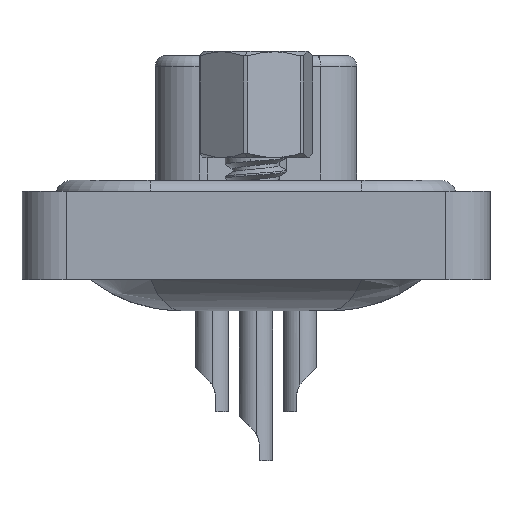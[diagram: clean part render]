
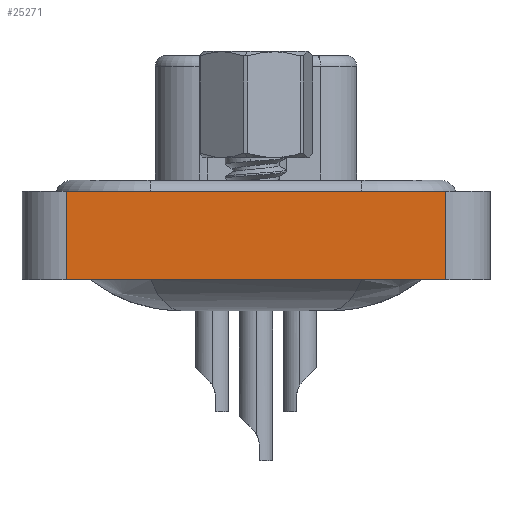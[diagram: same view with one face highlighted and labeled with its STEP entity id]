
A CAD part, left-side view. The second image highlights one B-rep face of the part: STEP entity #25271.
In plain terms, the highlighted planar face has unit normal (-1, 0, 0).
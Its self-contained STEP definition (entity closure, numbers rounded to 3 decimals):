
#2920 = AXIS2_PLACEMENT_3D ( 'NONE', #29742, #21012, #5306 ) ;
#4125 = VECTOR ( 'NONE', #22422, 1000. ) ;
#4745 = EDGE_CURVE ( 'NONE', #5199, #23662, #16815, .T. ) ;
#4768 = PLANE ( 'NONE',  #2920 ) ;
#5199 = VERTEX_POINT ( 'NONE', #11238 ) ;
#5306 = DIRECTION ( 'NONE',  ( 0., 0., 1. ) ) ;
#5752 = VECTOR ( 'NONE', #29520, 1000. ) ;
#6194 = DIRECTION ( 'NONE',  ( 0., 0., 1. ) ) ;
#6858 = ORIENTED_EDGE ( 'NONE', *, *, #12142, .T. ) ;
#8749 = CARTESIAN_POINT ( 'NONE',  ( -7.35, -8.55, 0.4 ) ) ;
#10289 = ORIENTED_EDGE ( 'NONE', *, *, #4745, .F. ) ;
#11238 = CARTESIAN_POINT ( 'NONE',  ( -7.35, 8.55, 0.4 ) ) ;
#12111 = CARTESIAN_POINT ( 'NONE',  ( -7.35, -8.55, -3.6 ) ) ;
#12142 = EDGE_CURVE ( 'NONE', #22488, #22613, #28128, .T. ) ;
#13203 = LINE ( 'NONE', #24951, #16382 ) ;
#13950 = CARTESIAN_POINT ( 'NONE',  ( -7.35, -8.55, 0.4 ) ) ;
#16382 = VECTOR ( 'NONE', #6194, 1000. ) ;
#16497 = EDGE_CURVE ( 'NONE', #22613, #23662, #18637, .T. ) ;
#16815 = LINE ( 'NONE', #13950, #32760 ) ;
#18637 = LINE ( 'NONE', #27011, #5752 ) ;
#20130 = ORIENTED_EDGE ( 'NONE', *, *, #16497, .T. ) ;
#21012 = DIRECTION ( 'NONE',  ( -1., 0., 0. ) ) ;
#22422 = DIRECTION ( 'NONE',  ( 0., -1., 0. ) ) ;
#22488 = VERTEX_POINT ( 'NONE', #32055 ) ;
#22613 = VERTEX_POINT ( 'NONE', #12111 ) ;
#23662 = VERTEX_POINT ( 'NONE', #8749 ) ;
#24951 = CARTESIAN_POINT ( 'NONE',  ( -7.35, 8.55, -3.6 ) ) ;
#25271 = ADVANCED_FACE ( 'NONE', ( #29046 ), #4768, .T. ) ;
#25455 = CARTESIAN_POINT ( 'NONE',  ( -7.35, -8.55, -3.6 ) ) ;
#26700 = ORIENTED_EDGE ( 'NONE', *, *, #30485, .F. ) ;
#27006 = EDGE_LOOP ( 'NONE', ( #20130, #10289, #26700, #6858 ) ) ;
#27011 = CARTESIAN_POINT ( 'NONE',  ( -7.35, -8.55, -3.6 ) ) ;
#28128 = LINE ( 'NONE', #25455, #4125 ) ;
#29046 = FACE_OUTER_BOUND ( 'NONE', #27006, .T. ) ;
#29520 = DIRECTION ( 'NONE',  ( 0., 0., 1. ) ) ;
#29742 = CARTESIAN_POINT ( 'NONE',  ( -7.35, -8.55, -3.6 ) ) ;
#30485 = EDGE_CURVE ( 'NONE', #22488, #5199, #13203, .T. ) ;
#32055 = CARTESIAN_POINT ( 'NONE',  ( -7.35, 8.55, -3.6 ) ) ;
#32760 = VECTOR ( 'NONE', #33220, 1000. ) ;
#33220 = DIRECTION ( 'NONE',  ( 0., -1., 0. ) ) ;
